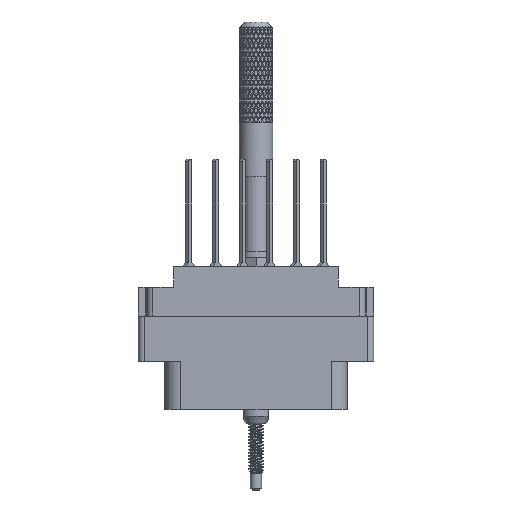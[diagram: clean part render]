
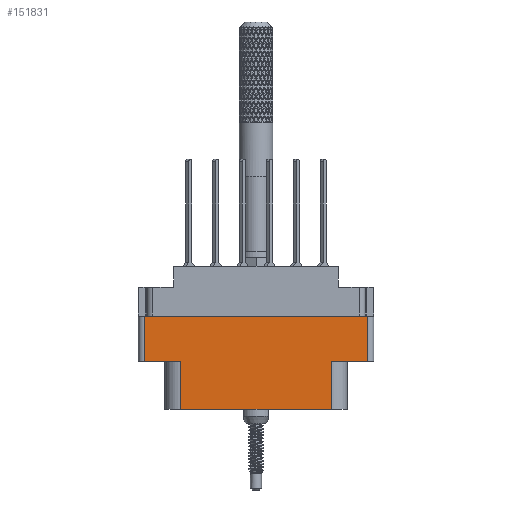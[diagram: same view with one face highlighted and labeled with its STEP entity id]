
A CAD part, front view. The second image highlights one B-rep face of the part: STEP entity #151831.
In plain terms, the highlighted planar face has unit normal (0, -1, 0).
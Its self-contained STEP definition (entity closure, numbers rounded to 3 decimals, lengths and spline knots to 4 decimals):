
#2992 = CARTESIAN_POINT ( 'NONE',  ( -0.624, -0.343, -0.798 ) ) ;
#7164 = CARTESIAN_POINT ( 'NONE',  ( 0.624, -0.343, -0.529 ) ) ;
#9300 = LINE ( 'NONE', #88030, #66834 ) ;
#16991 = CARTESIAN_POINT ( 'NONE',  ( -0.42, -0.343, -0.529 ) ) ;
#22637 = DIRECTION ( 'NONE',  ( 0., 0., 1. ) ) ;
#28447 = DIRECTION ( 'NONE',  ( 1., 0., 0. ) ) ;
#31625 = DIRECTION ( 'NONE',  ( 1., 0., 0. ) ) ;
#32367 = VECTOR ( 'NONE', #108322, 39.3701 ) ;
#41592 = VERTEX_POINT ( 'NONE', #178995 ) ;
#45182 = CARTESIAN_POINT ( 'NONE',  ( 0., -0.343, -0.529 ) ) ;
#45887 = EDGE_CURVE ( 'NONE', #41592, #46829, #116437, .T. ) ;
#46121 = VERTEX_POINT ( 'NONE', #7164 ) ;
#46829 = VERTEX_POINT ( 'NONE', #92865 ) ;
#49506 = ORIENTED_EDGE ( 'NONE', *, *, #45887, .F. ) ;
#49938 = VECTOR ( 'NONE', #178980, 39.3701 ) ;
#49984 = ORIENTED_EDGE ( 'NONE', *, *, #120502, .T. ) ;
#50114 = EDGE_CURVE ( 'NONE', #120432, #86693, #73608, .T. ) ;
#51817 = CARTESIAN_POINT ( 'NONE',  ( -0.624, -0.343, -0.529 ) ) ;
#52980 = CARTESIAN_POINT ( 'NONE',  ( -0.624, -0.343, -0.277 ) ) ;
#58108 = VECTOR ( 'NONE', #127638, 39.3701 ) ;
#63285 = VECTOR ( 'NONE', #22637, 39.3701 ) ;
#63476 = EDGE_CURVE ( 'NONE', #64430, #102685, #9300, .T. ) ;
#63694 = ORIENTED_EDGE ( 'NONE', *, *, #137745, .T. ) ;
#64430 = VERTEX_POINT ( 'NONE', #51817 ) ;
#66834 = VECTOR ( 'NONE', #31625, 39.3701 ) ;
#70014 = LINE ( 'NONE', #82901, #32367 ) ;
#73608 = LINE ( 'NONE', #155495, #58108 ) ;
#74824 = DIRECTION ( 'NONE',  ( 0., 0., -1. ) ) ;
#78529 = DIRECTION ( 'NONE',  ( 0., 0., 1. ) ) ;
#79309 = AXIS2_PLACEMENT_3D ( 'NONE', #2992, #144953, #74824 ) ;
#82901 = CARTESIAN_POINT ( 'NONE',  ( -0.42, -0.343, -0.529 ) ) ;
#86693 = VERTEX_POINT ( 'NONE', #174597 ) ;
#88030 = CARTESIAN_POINT ( 'NONE',  ( 0., -0.343, -0.529 ) ) ;
#92865 = CARTESIAN_POINT ( 'NONE',  ( 0.42, -0.343, -0.798 ) ) ;
#100473 = VECTOR ( 'NONE', #158529, 39.3701 ) ;
#102685 = VERTEX_POINT ( 'NONE', #16991 ) ;
#108322 = DIRECTION ( 'NONE',  ( 0., 0., -1. ) ) ;
#109931 = EDGE_CURVE ( 'NONE', #64430, #120432, #180860, .T. ) ;
#110192 = LINE ( 'NONE', #135608, #172266 ) ;
#115910 = LINE ( 'NONE', #45182, #100473 ) ;
#116437 = LINE ( 'NONE', #152946, #49938 ) ;
#120432 = VERTEX_POINT ( 'NONE', #52980 ) ;
#120502 = EDGE_CURVE ( 'NONE', #46121, #86693, #110192, .T. ) ;
#122361 = CARTESIAN_POINT ( 'NONE',  ( -0.624, -0.343, -0.798 ) ) ;
#127638 = DIRECTION ( 'NONE',  ( 1., 0., 0. ) ) ;
#128551 = ORIENTED_EDGE ( 'NONE', *, *, #50114, .F. ) ;
#131244 = EDGE_CURVE ( 'NONE', #102685, #153586, #70014, .T. ) ;
#133896 = EDGE_LOOP ( 'NONE', ( #137232, #63694, #49506, #156701, #49984, #128551, #155480, #165460 ) ) ;
#135608 = CARTESIAN_POINT ( 'NONE',  ( 0.624, -0.343, -0.798 ) ) ;
#136400 = EDGE_CURVE ( 'NONE', #46121, #41592, #115910, .T. ) ;
#137232 = ORIENTED_EDGE ( 'NONE', *, *, #131244, .T. ) ;
#137745 = EDGE_CURVE ( 'NONE', #153586, #46829, #149001, .T. ) ;
#142762 = CARTESIAN_POINT ( 'NONE',  ( -0.42, -0.343, -0.798 ) ) ;
#144953 = DIRECTION ( 'NONE',  ( 0., -1., 0. ) ) ;
#145620 = CARTESIAN_POINT ( 'NONE',  ( -0.624, -0.343, -0.798 ) ) ;
#149001 = LINE ( 'NONE', #145620, #171054 ) ;
#151831 = ADVANCED_FACE ( 'NONE', ( #155759 ), #160303, .T. ) ;
#152946 = CARTESIAN_POINT ( 'NONE',  ( 0.42, -0.343, -0.529 ) ) ;
#153586 = VERTEX_POINT ( 'NONE', #142762 ) ;
#155480 = ORIENTED_EDGE ( 'NONE', *, *, #109931, .F. ) ;
#155495 = CARTESIAN_POINT ( 'NONE',  ( -0.656, -0.343, -0.277 ) ) ;
#155759 = FACE_OUTER_BOUND ( 'NONE', #133896, .T. ) ;
#156701 = ORIENTED_EDGE ( 'NONE', *, *, #136400, .F. ) ;
#158529 = DIRECTION ( 'NONE',  ( -1., 0., 0. ) ) ;
#160303 = PLANE ( 'NONE',  #79309 ) ;
#165460 = ORIENTED_EDGE ( 'NONE', *, *, #63476, .T. ) ;
#171054 = VECTOR ( 'NONE', #28447, 39.3701 ) ;
#172266 = VECTOR ( 'NONE', #78529, 39.3701 ) ;
#174597 = CARTESIAN_POINT ( 'NONE',  ( 0.624, -0.343, -0.277 ) ) ;
#178980 = DIRECTION ( 'NONE',  ( 0., 0., -1. ) ) ;
#178995 = CARTESIAN_POINT ( 'NONE',  ( 0.42, -0.343, -0.529 ) ) ;
#180860 = LINE ( 'NONE', #122361, #63285 ) ;
